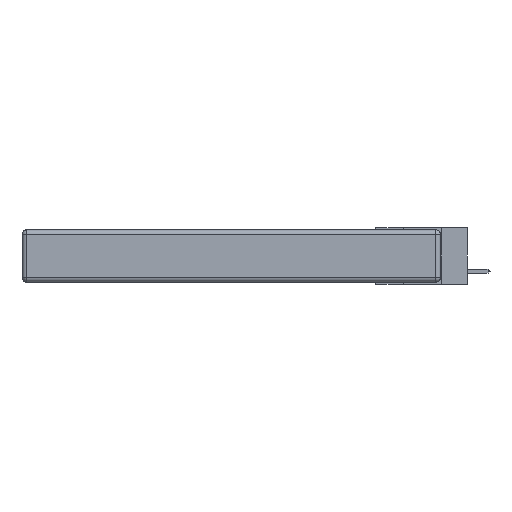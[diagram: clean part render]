
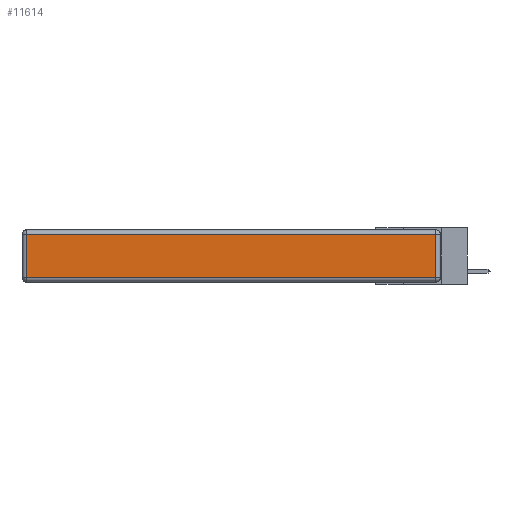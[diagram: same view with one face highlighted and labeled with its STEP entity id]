
A CAD part, left-side view. The second image highlights one B-rep face of the part: STEP entity #11614.
In plain terms, the highlighted planar face has unit normal (-1, 0, 0).
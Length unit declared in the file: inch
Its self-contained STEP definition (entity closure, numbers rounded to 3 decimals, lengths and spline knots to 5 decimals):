
#371 = ORIENTED_EDGE ( 'NONE', *, *, #8349, .T. ) ;
#1476 = CARTESIAN_POINT ( 'NONE',  ( 0., 2.72, -0.313 ) ) ;
#1620 = VERTEX_POINT ( 'NONE', #3019 ) ;
#1849 = EDGE_CURVE ( 'NONE', #2394, #9446, #5049, .T. ) ;
#2269 = VECTOR ( 'NONE', #3727, 39.37008 ) ;
#2394 = VERTEX_POINT ( 'NONE', #3112 ) ;
#3019 = CARTESIAN_POINT ( 'NONE',  ( 0., 0.03, -0.313 ) ) ;
#3112 = CARTESIAN_POINT ( 'NONE',  ( 0., 2.72, -0.03 ) ) ;
#3727 = DIRECTION ( 'NONE',  ( 0., 0., 1. ) ) ;
#3813 = VERTEX_POINT ( 'NONE', #5981 ) ;
#3894 = DIRECTION ( 'NONE',  ( 0., -1., 0. ) ) ;
#4666 = PLANE ( 'NONE',  #6804 ) ;
#5049 = LINE ( 'NONE', #7207, #20021 ) ;
#5570 = DIRECTION ( 'NONE',  ( 0., 1., 0. ) ) ;
#5768 = LINE ( 'NONE', #8492, #6721 ) ;
#5981 = CARTESIAN_POINT ( 'NONE',  ( 0., 0.03, -0.03 ) ) ;
#6160 = CARTESIAN_POINT ( 'NONE',  ( 0., 0., -0.343 ) ) ;
#6293 = EDGE_LOOP ( 'NONE', ( #12305, #16514, #371, #13207 ) ) ;
#6721 = VECTOR ( 'NONE', #3894, 39.37008 ) ;
#6804 = AXIS2_PLACEMENT_3D ( 'NONE', #6160, #10739, #16925 ) ;
#7207 = CARTESIAN_POINT ( 'NONE',  ( 0., 2.72, -0.343 ) ) ;
#7880 = EDGE_CURVE ( 'NONE', #1620, #3813, #15138, .T. ) ;
#8313 = CARTESIAN_POINT ( 'NONE',  ( 0., 0.03, -0.343 ) ) ;
#8349 = EDGE_CURVE ( 'NONE', #3813, #2394, #12900, .T. ) ;
#8492 = CARTESIAN_POINT ( 'NONE',  ( 0., 0., -0.313 ) ) ;
#9446 = VERTEX_POINT ( 'NONE', #1476 ) ;
#9612 = FACE_OUTER_BOUND ( 'NONE', #6293, .T. ) ;
#10739 = DIRECTION ( 'NONE',  ( -1., 0., 0. ) ) ;
#11115 = EDGE_CURVE ( 'NONE', #9446, #1620, #5768, .T. ) ;
#11614 = ADVANCED_FACE ( 'NONE', ( #9612 ), #4666, .T. ) ;
#12305 = ORIENTED_EDGE ( 'NONE', *, *, #11115, .T. ) ;
#12900 = LINE ( 'NONE', #19516, #19197 ) ;
#13207 = ORIENTED_EDGE ( 'NONE', *, *, #1849, .T. ) ;
#15138 = LINE ( 'NONE', #8313, #2269 ) ;
#16514 = ORIENTED_EDGE ( 'NONE', *, *, #7880, .T. ) ;
#16925 = DIRECTION ( 'NONE',  ( 0., 0., 1. ) ) ;
#18059 = DIRECTION ( 'NONE',  ( 0., 0., -1. ) ) ;
#19197 = VECTOR ( 'NONE', #5570, 39.37008 ) ;
#19516 = CARTESIAN_POINT ( 'NONE',  ( 0., 2.75, -0.03 ) ) ;
#20021 = VECTOR ( 'NONE', #18059, 39.37008 ) ;
